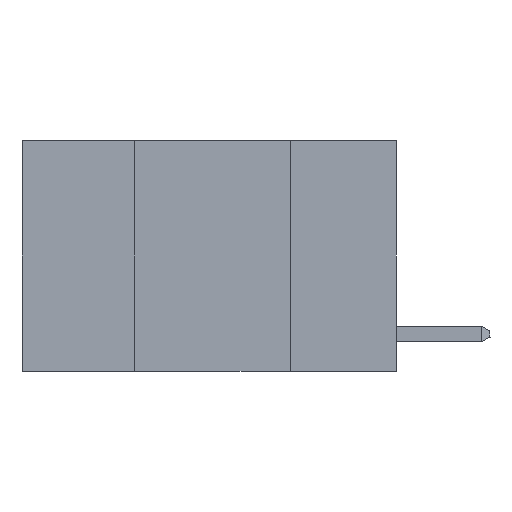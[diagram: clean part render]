
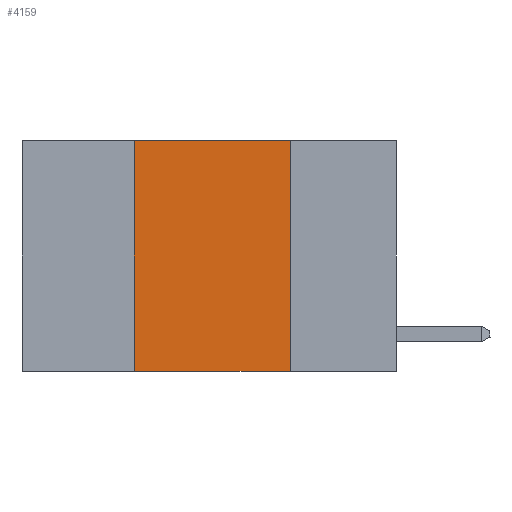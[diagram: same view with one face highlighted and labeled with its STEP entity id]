
A CAD part, left-side view. The second image highlights one B-rep face of the part: STEP entity #4159.
In plain terms, the highlighted planar face has unit normal (-1, 0, 0).
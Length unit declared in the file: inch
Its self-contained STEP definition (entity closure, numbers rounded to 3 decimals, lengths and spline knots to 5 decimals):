
#280 = VERTEX_POINT ( 'NONE', #9173 ) ;
#739 = EDGE_CURVE ( 'NONE', #12665, #13045, #12573, .T. ) ;
#2647 = CARTESIAN_POINT ( 'NONE',  ( 0., 0.6, 0. ) ) ;
#3494 = CARTESIAN_POINT ( 'NONE',  ( 0., 0.17, 0. ) ) ;
#3901 = DIRECTION ( 'NONE',  ( 0., -1., 0. ) ) ;
#4159 = ADVANCED_FACE ( 'NONE', ( #15810 ), #7205, .F. ) ;
#4419 = ORIENTED_EDGE ( 'NONE', *, *, #14708, .F. ) ;
#4565 = CARTESIAN_POINT ( 'NONE',  ( 0., 0.6, -0.37 ) ) ;
#4710 = DIRECTION ( 'NONE',  ( 0., 0., -1. ) ) ;
#7205 = PLANE ( 'NONE',  #9318 ) ;
#8346 = EDGE_CURVE ( 'NONE', #13045, #280, #15808, .T. ) ;
#8418 = DIRECTION ( 'NONE',  ( 0., 0., -1. ) ) ;
#8429 = ORIENTED_EDGE ( 'NONE', *, *, #739, .F. ) ;
#9173 = CARTESIAN_POINT ( 'NONE',  ( 0., 0.17, 0. ) ) ;
#9318 = AXIS2_PLACEMENT_3D ( 'NONE', #14545, #15722, #8418 ) ;
#9466 = CARTESIAN_POINT ( 'NONE',  ( 0., 0.17, -0.37 ) ) ;
#9666 = VECTOR ( 'NONE', #15054, 39.37008 ) ;
#9684 = CARTESIAN_POINT ( 'NONE',  ( 0., 0.42, 0. ) ) ;
#11272 = VECTOR ( 'NONE', #4710, 39.37008 ) ;
#11661 = LINE ( 'NONE', #3494, #11272 ) ;
#11753 = ORIENTED_EDGE ( 'NONE', *, *, #13539, .T. ) ;
#11946 = DIRECTION ( 'NONE',  ( 0., -1., 0. ) ) ;
#12259 = VECTOR ( 'NONE', #3901, 39.37008 ) ;
#12573 = LINE ( 'NONE', #14822, #9666 ) ;
#12665 = VERTEX_POINT ( 'NONE', #15107 ) ;
#12670 = VECTOR ( 'NONE', #11946, 39.37008 ) ;
#12905 = VERTEX_POINT ( 'NONE', #9466 ) ;
#13045 = VERTEX_POINT ( 'NONE', #9684 ) ;
#13047 = LINE ( 'NONE', #4565, #12670 ) ;
#13539 = EDGE_CURVE ( 'NONE', #12665, #12905, #13047, .T. ) ;
#14201 = ORIENTED_EDGE ( 'NONE', *, *, #8346, .F. ) ;
#14545 = CARTESIAN_POINT ( 'NONE',  ( 0., 0.6, 0. ) ) ;
#14708 = EDGE_CURVE ( 'NONE', #280, #12905, #11661, .T. ) ;
#14822 = CARTESIAN_POINT ( 'NONE',  ( 0., 0.42, 0. ) ) ;
#15054 = DIRECTION ( 'NONE',  ( 0., 0., 1. ) ) ;
#15107 = CARTESIAN_POINT ( 'NONE',  ( 0., 0.42, -0.37 ) ) ;
#15281 = EDGE_LOOP ( 'NONE', ( #4419, #14201, #8429, #11753 ) ) ;
#15722 = DIRECTION ( 'NONE',  ( 1., 0., 0. ) ) ;
#15808 = LINE ( 'NONE', #2647, #12259 ) ;
#15810 = FACE_OUTER_BOUND ( 'NONE', #15281, .T. ) ;
